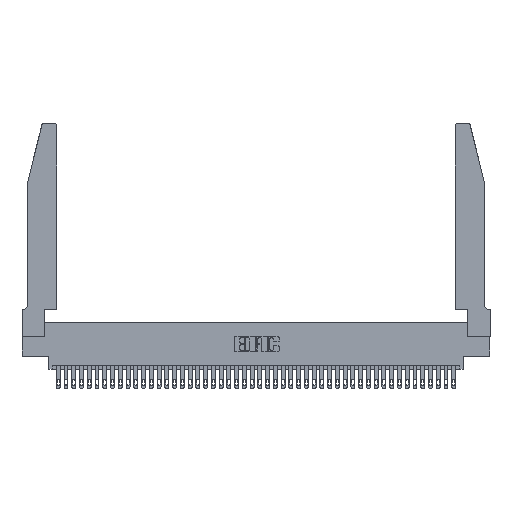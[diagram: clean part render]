
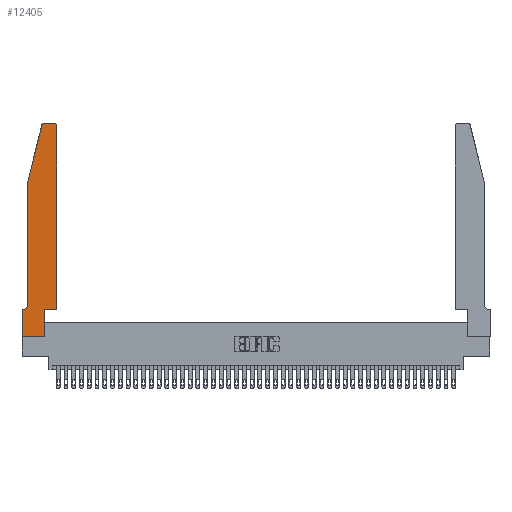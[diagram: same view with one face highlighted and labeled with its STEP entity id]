
A CAD part, top view. The second image highlights one B-rep face of the part: STEP entity #12405.
In plain terms, the highlighted planar face has unit normal (0, 0, 1).
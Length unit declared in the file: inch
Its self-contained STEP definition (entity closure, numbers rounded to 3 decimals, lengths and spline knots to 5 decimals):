
#462 = ORIENTED_EDGE ( 'NONE', *, *, #25202, .T. ) ;
#884 = CARTESIAN_POINT ( 'NONE',  ( 0.0755, 2., 0.37 ) ) ;
#2053 = VERTEX_POINT ( 'NONE', #43056 ) ;
#2313 = CARTESIAN_POINT ( 'NONE',  ( 0.4505, 0.35, 0.37 ) ) ;
#2576 = CARTESIAN_POINT ( 'NONE',  ( 0., 0., 0.37 ) ) ;
#2916 = DIRECTION ( 'NONE',  ( -1., 0., 0. ) ) ;
#3143 = DIRECTION ( 'NONE',  ( 1., 0., 0. ) ) ;
#3441 = DIRECTION ( 'NONE',  ( 0., 0., 1. ) ) ;
#3627 = CARTESIAN_POINT ( 'NONE',  ( 0.4505, 0.35, 0.37 ) ) ;
#3690 = PLANE ( 'NONE',  #27749 ) ;
#3722 = LINE ( 'NONE', #3627, #31609 ) ;
#4140 = CIRCLE ( 'NONE', #17342, 0.03 ) ;
#4349 = EDGE_CURVE ( 'NONE', #12645, #19228, #24474, .T. ) ;
#4426 = CARTESIAN_POINT ( 'NONE',  ( 0., 0., 0.37 ) ) ;
#5234 = EDGE_LOOP ( 'NONE', ( #8878, #35917, #41125, #462, #32717, #12633, #13911, #18387, #34704, #37783, #43372, #17395 ) ) ;
#5454 = AXIS2_PLACEMENT_3D ( 'NONE', #21752, #22072, #18615 ) ;
#6271 = VECTOR ( 'NONE', #21636, 39.37008 ) ;
#6496 = VECTOR ( 'NONE', #18794, 39.37008 ) ;
#6981 = DIRECTION ( 'NONE',  ( 1., 0., 0. ) ) ;
#7217 = EDGE_CURVE ( 'NONE', #34361, #18848, #3722, .T. ) ;
#7931 = CIRCLE ( 'NONE', #5454, 0.07 ) ;
#8540 = EDGE_CURVE ( 'NONE', #39649, #33252, #7931, .T. ) ;
#8878 = ORIENTED_EDGE ( 'NONE', *, *, #27586, .T. ) ;
#10543 = CARTESIAN_POINT ( 'NONE',  ( 0., 0.35, 0.37 ) ) ;
#10670 = CARTESIAN_POINT ( 'NONE',  ( 0., 0.35, 0.37 ) ) ;
#11147 = DIRECTION ( 'NONE',  ( 1., 0., 0. ) ) ;
#11186 = VECTOR ( 'NONE', #17766, 39.37008 ) ;
#11465 = DIRECTION ( 'NONE',  ( 0., 0., 1. ) ) ;
#12405 = ADVANCED_FACE ( 'NONE', ( #15171 ), #3690, .T. ) ;
#12633 = ORIENTED_EDGE ( 'NONE', *, *, #28056, .T. ) ;
#12645 = VERTEX_POINT ( 'NONE', #30358 ) ;
#13202 = LINE ( 'NONE', #2576, #14258 ) ;
#13377 = CARTESIAN_POINT ( 'NONE',  ( 0.2865, 0.35, 0.37 ) ) ;
#13736 = LINE ( 'NONE', #27804, #40051 ) ;
#13853 = CARTESIAN_POINT ( 'NONE',  ( 0.4205, 2.72, 0.37 ) ) ;
#13911 = ORIENTED_EDGE ( 'NONE', *, *, #25800, .T. ) ;
#14258 = VECTOR ( 'NONE', #3143, 39.37008 ) ;
#15171 = FACE_OUTER_BOUND ( 'NONE', #5234, .T. ) ;
#15575 = LINE ( 'NONE', #4426, #6496 ) ;
#17288 = DIRECTION ( 'NONE',  ( 1., 0., 0. ) ) ;
#17342 = AXIS2_PLACEMENT_3D ( 'NONE', #42147, #11465, #11147 ) ;
#17395 = ORIENTED_EDGE ( 'NONE', *, *, #39583, .T. ) ;
#17448 = EDGE_CURVE ( 'NONE', #18848, #24923, #23363, .T. ) ;
#17766 = DIRECTION ( 'NONE',  ( 0., 1., 0. ) ) ;
#18055 = CARTESIAN_POINT ( 'NONE',  ( 0., 0., 0.37 ) ) ;
#18387 = ORIENTED_EDGE ( 'NONE', *, *, #39377, .T. ) ;
#18615 = DIRECTION ( 'NONE',  ( -1., 0., 0. ) ) ;
#18794 = DIRECTION ( 'NONE',  ( 0., -1., 0. ) ) ;
#18848 = VERTEX_POINT ( 'NONE', #2313 ) ;
#19228 = VERTEX_POINT ( 'NONE', #884 ) ;
#21636 = DIRECTION ( 'NONE',  ( -0.239, -0.971, 0. ) ) ;
#21752 = CARTESIAN_POINT ( 'NONE',  ( 0.0055, 0.42, 0.37 ) ) ;
#22072 = DIRECTION ( 'NONE',  ( 0., 0., -1. ) ) ;
#23113 = LINE ( 'NONE', #43214, #41826 ) ;
#23363 = LINE ( 'NONE', #29217, #28730 ) ;
#23370 = VECTOR ( 'NONE', #2916, 39.37008 ) ;
#23394 = CARTESIAN_POINT ( 'NONE',  ( 0.0055, 0.35, 0.37 ) ) ;
#24474 = LINE ( 'NONE', #25111, #6271 ) ;
#24825 = CARTESIAN_POINT ( 'NONE',  ( 0.2865, 0.35, 0.37 ) ) ;
#24923 = VERTEX_POINT ( 'NONE', #40872 ) ;
#24951 = LINE ( 'NONE', #36890, #23370 ) ;
#24966 = AXIS2_PLACEMENT_3D ( 'NONE', #13853, #3441, #41119 ) ;
#25111 = CARTESIAN_POINT ( 'NONE',  ( 0.0755, 2., 0.37 ) ) ;
#25202 = EDGE_CURVE ( 'NONE', #19228, #39649, #23113, .T. ) ;
#25800 = EDGE_CURVE ( 'NONE', #40248, #31973, #15575, .T. ) ;
#26899 = CARTESIAN_POINT ( 'NONE',  ( 0.2865, 0., 0.37 ) ) ;
#27586 = EDGE_CURVE ( 'NONE', #38150, #2053, #13736, .T. ) ;
#27749 = AXIS2_PLACEMENT_3D ( 'NONE', #10543, #37679, #6981 ) ;
#27804 = CARTESIAN_POINT ( 'NONE',  ( 0.2605, 2.75, 0.37 ) ) ;
#28038 = VERTEX_POINT ( 'NONE', #26899 ) ;
#28056 = EDGE_CURVE ( 'NONE', #33252, #40248, #24951, .T. ) ;
#28730 = VECTOR ( 'NONE', #32189, 39.37008 ) ;
#29217 = CARTESIAN_POINT ( 'NONE',  ( 0.4505, 0.35, 0.37 ) ) ;
#30358 = CARTESIAN_POINT ( 'NONE',  ( 0.25487, 2.72718, 0.37 ) ) ;
#31609 = VECTOR ( 'NONE', #17288, 39.37008 ) ;
#31973 = VERTEX_POINT ( 'NONE', #18055 ) ;
#32117 = EDGE_CURVE ( 'NONE', #28038, #34361, #35898, .T. ) ;
#32189 = DIRECTION ( 'NONE',  ( 0., 1., 0. ) ) ;
#32717 = ORIENTED_EDGE ( 'NONE', *, *, #8540, .T. ) ;
#33252 = VERTEX_POINT ( 'NONE', #23394 ) ;
#34042 = EDGE_CURVE ( 'NONE', #2053, #12645, #4140, .T. ) ;
#34361 = VERTEX_POINT ( 'NONE', #13377 ) ;
#34704 = ORIENTED_EDGE ( 'NONE', *, *, #32117, .T. ) ;
#35708 = CIRCLE ( 'NONE', #24966, 0.03 ) ;
#35898 = LINE ( 'NONE', #24825, #11186 ) ;
#35917 = ORIENTED_EDGE ( 'NONE', *, *, #34042, .T. ) ;
#36319 = CARTESIAN_POINT ( 'NONE',  ( 0.4205, 2.75, 0.37 ) ) ;
#36890 = CARTESIAN_POINT ( 'NONE',  ( 0.0755, 0.35, 0.37 ) ) ;
#37679 = DIRECTION ( 'NONE',  ( 0., 0., 1. ) ) ;
#37783 = ORIENTED_EDGE ( 'NONE', *, *, #7217, .T. ) ;
#38111 = DIRECTION ( 'NONE',  ( -1., 0., 0. ) ) ;
#38150 = VERTEX_POINT ( 'NONE', #36319 ) ;
#39377 = EDGE_CURVE ( 'NONE', #31973, #28038, #13202, .T. ) ;
#39583 = EDGE_CURVE ( 'NONE', #24923, #38150, #35708, .T. ) ;
#39649 = VERTEX_POINT ( 'NONE', #41844 ) ;
#39821 = DIRECTION ( 'NONE',  ( 0., -1., 0. ) ) ;
#40051 = VECTOR ( 'NONE', #38111, 39.37008 ) ;
#40248 = VERTEX_POINT ( 'NONE', #10670 ) ;
#40872 = CARTESIAN_POINT ( 'NONE',  ( 0.4505, 2.72, 0.37 ) ) ;
#41119 = DIRECTION ( 'NONE',  ( 1., 0., 0. ) ) ;
#41125 = ORIENTED_EDGE ( 'NONE', *, *, #4349, .T. ) ;
#41826 = VECTOR ( 'NONE', #39821, 39.37008 ) ;
#41844 = CARTESIAN_POINT ( 'NONE',  ( 0.0755, 0.42, 0.37 ) ) ;
#42147 = CARTESIAN_POINT ( 'NONE',  ( 0.284, 2.72, 0.37 ) ) ;
#43056 = CARTESIAN_POINT ( 'NONE',  ( 0.284, 2.75, 0.37 ) ) ;
#43214 = CARTESIAN_POINT ( 'NONE',  ( 0.0755, 2., 0.37 ) ) ;
#43372 = ORIENTED_EDGE ( 'NONE', *, *, #17448, .T. ) ;
